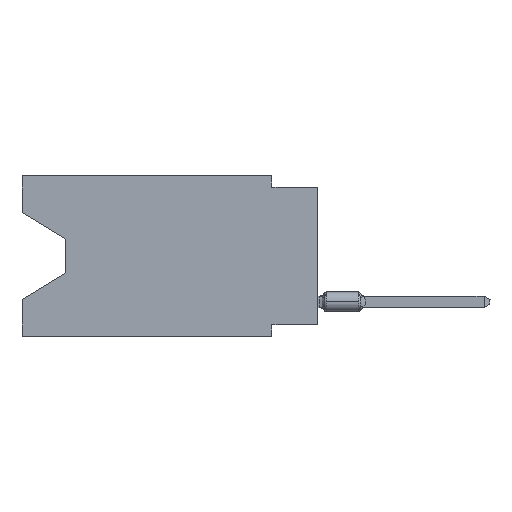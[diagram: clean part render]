
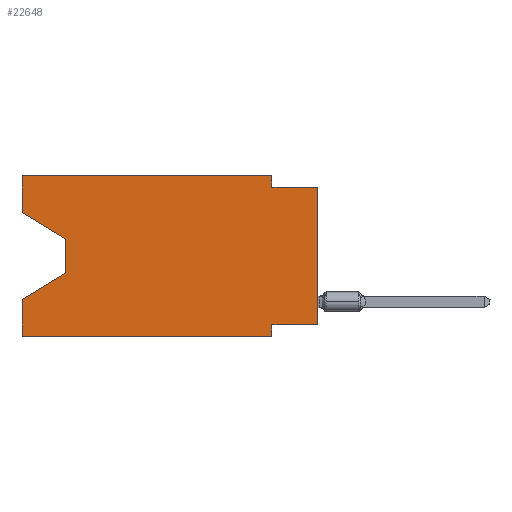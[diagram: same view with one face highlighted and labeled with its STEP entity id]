
A CAD part, left-side view. The second image highlights one B-rep face of the part: STEP entity #22648.
In plain terms, the highlighted planar face has unit normal (-1, 0, 0).
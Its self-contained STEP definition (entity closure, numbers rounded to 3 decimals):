
#136 = VECTOR ( 'NONE', #47361, 1000. ) ;
#205 = LINE ( 'NONE', #50383, #22769 ) ;
#297 = CARTESIAN_POINT ( 'NONE',  ( 0., 16.383, -8.89 ) ) ;
#401 = CARTESIAN_POINT ( 'NONE',  ( 0., 0., -0.635 ) ) ;
#670 = LINE ( 'NONE', #401, #48158 ) ;
#1158 = VECTOR ( 'NONE', #5354, 1000. ) ;
#1558 = CARTESIAN_POINT ( 'NONE',  ( 0., 0., -8.255 ) ) ;
#1780 = CARTESIAN_POINT ( 'NONE',  ( 0., 16.383, 0. ) ) ;
#1793 = VERTEX_POINT ( 'NONE', #52899 ) ;
#1986 = ORIENTED_EDGE ( 'NONE', *, *, #6786, .T. ) ;
#3168 = CARTESIAN_POINT ( 'NONE',  ( 0., 2.54, -0.635 ) ) ;
#4217 = EDGE_CURVE ( 'NONE', #6467, #6848, #205, .T. ) ;
#4391 = EDGE_CURVE ( 'NONE', #53984, #25002, #13910, .T. ) ;
#4406 = DIRECTION ( 'NONE',  ( 1., 0., 0. ) ) ;
#4469 = CARTESIAN_POINT ( 'NONE',  ( 0., 0., -8.255 ) ) ;
#4566 = ORIENTED_EDGE ( 'NONE', *, *, #4217, .F. ) ;
#4702 = ORIENTED_EDGE ( 'NONE', *, *, #53565, .F. ) ;
#4880 = CARTESIAN_POINT ( 'NONE',  ( 0., 13.97, -5.385 ) ) ;
#5059 = CARTESIAN_POINT ( 'NONE',  ( 0., 16.383, -8.89 ) ) ;
#5354 = DIRECTION ( 'NONE',  ( 0., 0., -1. ) ) ;
#5609 = DIRECTION ( 'NONE',  ( 0., -1., 0. ) ) ;
#5767 = VECTOR ( 'NONE', #20698, 1000. ) ;
#6048 = VERTEX_POINT ( 'NONE', #16472 ) ;
#6122 = CARTESIAN_POINT ( 'NONE',  ( 0., 13.97, -3.505 ) ) ;
#6429 = CARTESIAN_POINT ( 'NONE',  ( 0., 2.54, 0. ) ) ;
#6467 = VERTEX_POINT ( 'NONE', #38932 ) ;
#6786 = EDGE_CURVE ( 'NONE', #53984, #1793, #31442, .T. ) ;
#6788 = ORIENTED_EDGE ( 'NONE', *, *, #41639, .F. ) ;
#6848 = VERTEX_POINT ( 'NONE', #10608 ) ;
#6976 = LINE ( 'NONE', #23716, #49756 ) ;
#7409 = DIRECTION ( 'NONE',  ( 0., 0., -1. ) ) ;
#7875 = VECTOR ( 'NONE', #18314, 1000. ) ;
#9857 = EDGE_CURVE ( 'NONE', #34975, #15328, #47840, .T. ) ;
#9912 = ORIENTED_EDGE ( 'NONE', *, *, #12675, .T. ) ;
#10608 = CARTESIAN_POINT ( 'NONE',  ( 0., 2.54, 0. ) ) ;
#12675 = EDGE_CURVE ( 'NONE', #41252, #15485, #24258, .T. ) ;
#13555 = DIRECTION ( 'NONE',  ( 0., 0., -1. ) ) ;
#13910 = LINE ( 'NONE', #1558, #7875 ) ;
#15142 = ORIENTED_EDGE ( 'NONE', *, *, #4391, .F. ) ;
#15328 = VERTEX_POINT ( 'NONE', #25360 ) ;
#15485 = VERTEX_POINT ( 'NONE', #18887 ) ;
#15497 = VECTOR ( 'NONE', #47378, 1000. ) ;
#16472 = CARTESIAN_POINT ( 'NONE',  ( 0., 13.97, -5.385 ) ) ;
#17141 = LINE ( 'NONE', #5059, #34087 ) ;
#17365 = EDGE_CURVE ( 'NONE', #6048, #15328, #30645, .T. ) ;
#17602 = VECTOR ( 'NONE', #23926, 1000. ) ;
#18314 = DIRECTION ( 'NONE',  ( 0., 1., 0. ) ) ;
#18320 = EDGE_CURVE ( 'NONE', #41252, #6467, #6976, .T. ) ;
#18887 = CARTESIAN_POINT ( 'NONE',  ( 0., 13.97, -3.505 ) ) ;
#19685 = ORIENTED_EDGE ( 'NONE', *, *, #21887, .F. ) ;
#19855 = DIRECTION ( 'NONE',  ( 0., 0., 1. ) ) ;
#20698 = DIRECTION ( 'NONE',  ( 0., -0.855, -0.519 ) ) ;
#21135 = PLANE ( 'NONE',  #39479 ) ;
#21887 = EDGE_CURVE ( 'NONE', #45972, #1793, #670, .T. ) ;
#22648 = ADVANCED_FACE ( 'NONE', ( #44982 ), #21135, .F. ) ;
#22696 = CARTESIAN_POINT ( 'NONE',  ( 0., 0., 0. ) ) ;
#22715 = ORIENTED_EDGE ( 'NONE', *, *, #50869, .T. ) ;
#22769 = VECTOR ( 'NONE', #50118, 1000. ) ;
#23716 = CARTESIAN_POINT ( 'NONE',  ( 0., 16.383, 0. ) ) ;
#23926 = DIRECTION ( 'NONE',  ( 0., 0., -1. ) ) ;
#24258 = LINE ( 'NONE', #48942, #5767 ) ;
#25002 = VERTEX_POINT ( 'NONE', #48020 ) ;
#25360 = CARTESIAN_POINT ( 'NONE',  ( 0., 16.383, -6.852 ) ) ;
#30645 = LINE ( 'NONE', #4880, #15497 ) ;
#30949 = CARTESIAN_POINT ( 'NONE',  ( 0., 2.54, -8.89 ) ) ;
#31442 = LINE ( 'NONE', #22696, #136 ) ;
#32661 = ORIENTED_EDGE ( 'NONE', *, *, #53590, .T. ) ;
#34087 = VECTOR ( 'NONE', #5609, 1000. ) ;
#34975 = VERTEX_POINT ( 'NONE', #297 ) ;
#38932 = CARTESIAN_POINT ( 'NONE',  ( 0., 16.383, 0. ) ) ;
#39350 = VECTOR ( 'NONE', #13555, 1000. ) ;
#39479 = AXIS2_PLACEMENT_3D ( 'NONE', #46065, #4406, #7409 ) ;
#40244 = ORIENTED_EDGE ( 'NONE', *, *, #18320, .F. ) ;
#41252 = VERTEX_POINT ( 'NONE', #42492 ) ;
#41639 = EDGE_CURVE ( 'NONE', #6848, #45972, #51679, .T. ) ;
#42079 = ORIENTED_EDGE ( 'NONE', *, *, #9857, .F. ) ;
#42359 = DIRECTION ( 'NONE',  ( 0., -1., 0. ) ) ;
#42492 = CARTESIAN_POINT ( 'NONE',  ( 0., 16.383, -2.038 ) ) ;
#43466 = ORIENTED_EDGE ( 'NONE', *, *, #17365, .T. ) ;
#44982 = FACE_OUTER_BOUND ( 'NONE', #46568, .T. ) ;
#45972 = VERTEX_POINT ( 'NONE', #3168 ) ;
#46065 = CARTESIAN_POINT ( 'NONE',  ( 0., 16.383, 0. ) ) ;
#46568 = EDGE_LOOP ( 'NONE', ( #9912, #22715, #43466, #42079, #32661, #4702, #15142, #1986, #19685, #6788, #4566, #40244 ) ) ;
#47361 = DIRECTION ( 'NONE',  ( 0., 0., 1. ) ) ;
#47378 = DIRECTION ( 'NONE',  ( 0., 0.855, -0.519 ) ) ;
#47840 = LINE ( 'NONE', #1780, #49407 ) ;
#48020 = CARTESIAN_POINT ( 'NONE',  ( 0., 2.54, -8.255 ) ) ;
#48158 = VECTOR ( 'NONE', #42359, 1000. ) ;
#48942 = CARTESIAN_POINT ( 'NONE',  ( 0., 16.383, -2.038 ) ) ;
#49407 = VECTOR ( 'NONE', #52496, 1000. ) ;
#49756 = VECTOR ( 'NONE', #19855, 1000. ) ;
#50118 = DIRECTION ( 'NONE',  ( 0., -1., 0. ) ) ;
#50153 = VERTEX_POINT ( 'NONE', #30949 ) ;
#50383 = CARTESIAN_POINT ( 'NONE',  ( 0., 16.383, 0. ) ) ;
#50573 = CARTESIAN_POINT ( 'NONE',  ( 0., 2.54, -8.89 ) ) ;
#50869 = EDGE_CURVE ( 'NONE', #15485, #6048, #52980, .T. ) ;
#51666 = LINE ( 'NONE', #50573, #39350 ) ;
#51679 = LINE ( 'NONE', #6429, #1158 ) ;
#52496 = DIRECTION ( 'NONE',  ( 0., 0., 1. ) ) ;
#52899 = CARTESIAN_POINT ( 'NONE',  ( 0., 0., -0.635 ) ) ;
#52980 = LINE ( 'NONE', #6122, #17602 ) ;
#53565 = EDGE_CURVE ( 'NONE', #25002, #50153, #51666, .T. ) ;
#53590 = EDGE_CURVE ( 'NONE', #34975, #50153, #17141, .T. ) ;
#53984 = VERTEX_POINT ( 'NONE', #4469 ) ;
